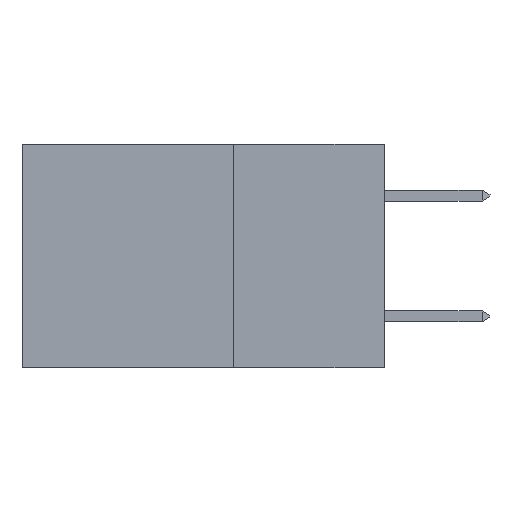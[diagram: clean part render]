
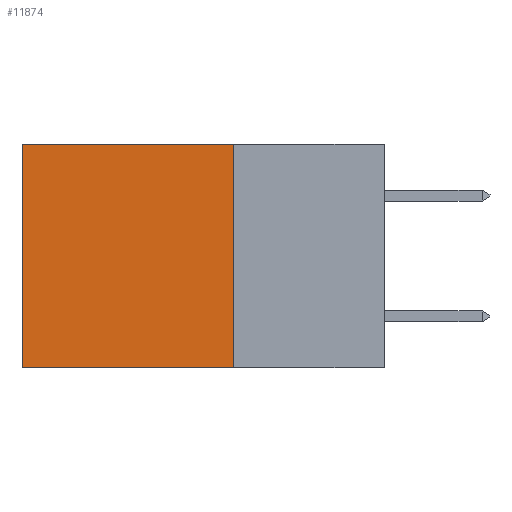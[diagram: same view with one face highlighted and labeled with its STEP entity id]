
A CAD part, left-side view. The second image highlights one B-rep face of the part: STEP entity #11874.
In plain terms, the highlighted planar face has unit normal (-1, 0, 0).
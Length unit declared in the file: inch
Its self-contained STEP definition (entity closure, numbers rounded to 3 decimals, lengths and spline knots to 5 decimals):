
#641 = DIRECTION ( 'NONE',  ( 0., 0., -1. ) ) ;
#1071 = ORIENTED_EDGE ( 'NONE', *, *, #3698, .F. ) ;
#1748 = VECTOR ( 'NONE', #641, 39.37008 ) ;
#1944 = ORIENTED_EDGE ( 'NONE', *, *, #4459, .T. ) ;
#1946 = CARTESIAN_POINT ( 'NONE',  ( 0.2875, 0.25, -0.37 ) ) ;
#2720 = CARTESIAN_POINT ( 'NONE',  ( 0.2875, 0.25, 0. ) ) ;
#3174 = ORIENTED_EDGE ( 'NONE', *, *, #10899, .F. ) ;
#3698 = EDGE_CURVE ( 'NONE', #19462, #9568, #20064, .T. ) ;
#3710 = CARTESIAN_POINT ( 'NONE',  ( 0.2875, 0.6, 0. ) ) ;
#3822 = CARTESIAN_POINT ( 'NONE',  ( 0.2875, 0.25, 0. ) ) ;
#3895 = DIRECTION ( 'NONE',  ( 0., 1., 0. ) ) ;
#3996 = VERTEX_POINT ( 'NONE', #19232 ) ;
#4459 = EDGE_CURVE ( 'NONE', #3996, #9568, #18530, .T. ) ;
#5797 = PLANE ( 'NONE',  #6336 ) ;
#5983 = FACE_OUTER_BOUND ( 'NONE', #14887, .T. ) ;
#6336 = AXIS2_PLACEMENT_3D ( 'NONE', #2720, #7528, #7457 ) ;
#7169 = VECTOR ( 'NONE', #16721, 39.37008 ) ;
#7457 = DIRECTION ( 'NONE',  ( 0., 0., -1. ) ) ;
#7528 = DIRECTION ( 'NONE',  ( 1., 0., 0. ) ) ;
#8089 = LINE ( 'NONE', #3822, #16380 ) ;
#8203 = ORIENTED_EDGE ( 'NONE', *, *, #14481, .T. ) ;
#9398 = LINE ( 'NONE', #11813, #13516 ) ;
#9568 = VERTEX_POINT ( 'NONE', #13254 ) ;
#10899 = EDGE_CURVE ( 'NONE', #20961, #19462, #9398, .T. ) ;
#11813 = CARTESIAN_POINT ( 'NONE',  ( 0.2875, 0.25, 0. ) ) ;
#11874 = ADVANCED_FACE ( 'NONE', ( #5983 ), #5797, .F. ) ;
#12581 = CARTESIAN_POINT ( 'NONE',  ( 0.2875, 0.25, 0. ) ) ;
#13254 = CARTESIAN_POINT ( 'NONE',  ( 0.2875, 0.6, -0.37 ) ) ;
#13516 = VECTOR ( 'NONE', #18196, 39.37008 ) ;
#14481 = EDGE_CURVE ( 'NONE', #20961, #3996, #8089, .T. ) ;
#14887 = EDGE_LOOP ( 'NONE', ( #1944, #1071, #3174, #8203 ) ) ;
#15677 = CARTESIAN_POINT ( 'NONE',  ( 0.2875, 0.25, -0.37 ) ) ;
#16380 = VECTOR ( 'NONE', #3895, 39.37008 ) ;
#16721 = DIRECTION ( 'NONE',  ( 0., 1., 0. ) ) ;
#18196 = DIRECTION ( 'NONE',  ( 0., 0., -1. ) ) ;
#18530 = LINE ( 'NONE', #3710, #1748 ) ;
#19232 = CARTESIAN_POINT ( 'NONE',  ( 0.2875, 0.6, 0. ) ) ;
#19462 = VERTEX_POINT ( 'NONE', #15677 ) ;
#20064 = LINE ( 'NONE', #1946, #7169 ) ;
#20961 = VERTEX_POINT ( 'NONE', #12581 ) ;
